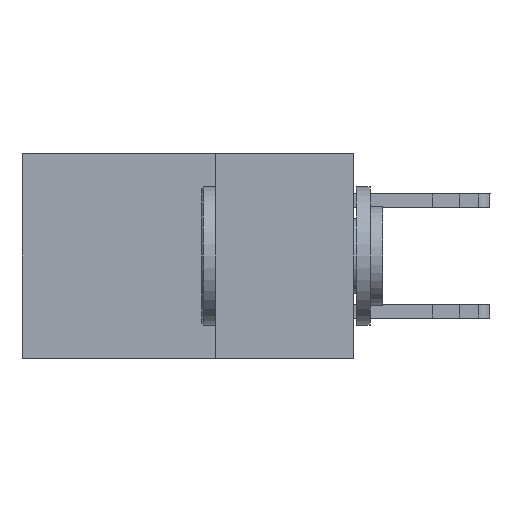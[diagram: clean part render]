
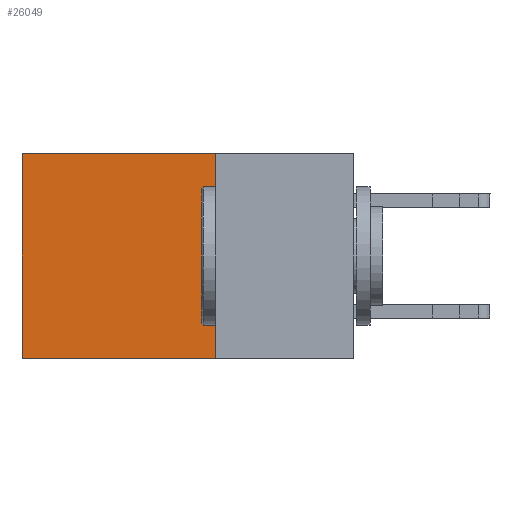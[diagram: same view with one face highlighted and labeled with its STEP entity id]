
A CAD part, left-side view. The second image highlights one B-rep face of the part: STEP entity #26049.
In plain terms, the highlighted planar face has unit normal (-1, 0, 0).
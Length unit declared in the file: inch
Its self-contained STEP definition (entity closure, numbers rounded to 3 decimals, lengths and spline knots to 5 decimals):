
#1092 = ORIENTED_EDGE ( 'NONE', *, *, #1292, .F. ) ;
#1205 = DIRECTION ( 'NONE',  ( 0., 1., 0. ) ) ;
#1292 = EDGE_CURVE ( 'NONE', #27835, #7553, #24463, .T. ) ;
#1324 = CARTESIAN_POINT ( 'NONE',  ( 0.2875, 0.25, -0.37 ) ) ;
#1481 = LINE ( 'NONE', #11891, #9642 ) ;
#3999 = VERTEX_POINT ( 'NONE', #31290 ) ;
#5086 = EDGE_LOOP ( 'NONE', ( #31792, #9913, #1092, #18166 ) ) ;
#7159 = CARTESIAN_POINT ( 'NONE',  ( 0.2875, 0.6, 0. ) ) ;
#7553 = VERTEX_POINT ( 'NONE', #15918 ) ;
#9233 = EDGE_CURVE ( 'NONE', #7553, #30940, #28797, .T. ) ;
#9642 = VECTOR ( 'NONE', #20269, 39.37008 ) ;
#9913 = ORIENTED_EDGE ( 'NONE', *, *, #9233, .F. ) ;
#10711 = PLANE ( 'NONE',  #18184 ) ;
#11891 = CARTESIAN_POINT ( 'NONE',  ( 0.2875, 0.25, 0. ) ) ;
#12051 = VECTOR ( 'NONE', #1205, 39.37008 ) ;
#13344 = CARTESIAN_POINT ( 'NONE',  ( 0.2875, 0.25, 0. ) ) ;
#15041 = DIRECTION ( 'NONE',  ( 0., 0., -1. ) ) ;
#15918 = CARTESIAN_POINT ( 'NONE',  ( 0.2875, 0.25, -0.37 ) ) ;
#16092 = DIRECTION ( 'NONE',  ( 0., 0., -1. ) ) ;
#16279 = CARTESIAN_POINT ( 'NONE',  ( 0.2875, 0.25, 0. ) ) ;
#18166 = ORIENTED_EDGE ( 'NONE', *, *, #28269, .T. ) ;
#18184 = AXIS2_PLACEMENT_3D ( 'NONE', #13344, #24512, #16092 ) ;
#18368 = VECTOR ( 'NONE', #15041, 39.37008 ) ;
#19204 = FACE_OUTER_BOUND ( 'NONE', #5086, .T. ) ;
#20269 = DIRECTION ( 'NONE',  ( 0., 1., 0. ) ) ;
#24463 = LINE ( 'NONE', #16279, #33493 ) ;
#24512 = DIRECTION ( 'NONE',  ( 1., 0., 0. ) ) ;
#26049 = ADVANCED_FACE ( 'NONE', ( #19204 ), #10711, .F. ) ;
#27156 = CARTESIAN_POINT ( 'NONE',  ( 0.2875, 0.25, 0. ) ) ;
#27835 = VERTEX_POINT ( 'NONE', #27156 ) ;
#28269 = EDGE_CURVE ( 'NONE', #27835, #3999, #1481, .T. ) ;
#28797 = LINE ( 'NONE', #1324, #12051 ) ;
#30013 = LINE ( 'NONE', #7159, #18368 ) ;
#30940 = VERTEX_POINT ( 'NONE', #33595 ) ;
#31290 = CARTESIAN_POINT ( 'NONE',  ( 0.2875, 0.6, 0. ) ) ;
#31792 = ORIENTED_EDGE ( 'NONE', *, *, #31829, .T. ) ;
#31829 = EDGE_CURVE ( 'NONE', #3999, #30940, #30013, .T. ) ;
#33493 = VECTOR ( 'NONE', #35499, 39.37008 ) ;
#33595 = CARTESIAN_POINT ( 'NONE',  ( 0.2875, 0.6, -0.37 ) ) ;
#35499 = DIRECTION ( 'NONE',  ( 0., 0., -1. ) ) ;
